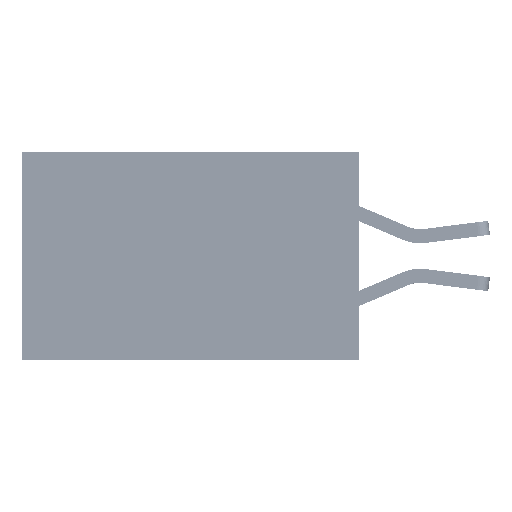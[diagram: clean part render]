
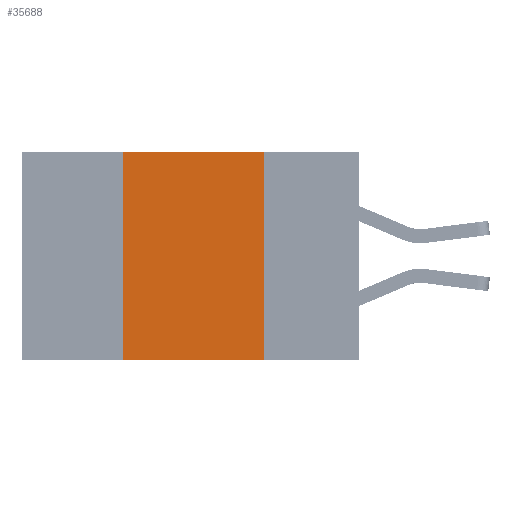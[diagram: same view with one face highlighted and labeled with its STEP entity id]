
A CAD part, left-side view. The second image highlights one B-rep face of the part: STEP entity #35688.
In plain terms, the highlighted planar face has unit normal (-1, 0, 0).
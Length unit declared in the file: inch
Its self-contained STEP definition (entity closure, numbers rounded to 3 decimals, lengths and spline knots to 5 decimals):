
#86 = VERTEX_POINT ( 'NONE', #17594 ) ;
#733 = DIRECTION ( 'NONE',  ( 0., -1., 0. ) ) ;
#2253 = LINE ( 'NONE', #8160, #23089 ) ;
#2528 = DIRECTION ( 'NONE',  ( 0., -1., 0. ) ) ;
#2641 = LINE ( 'NONE', #4090, #31487 ) ;
#4090 = CARTESIAN_POINT ( 'NONE',  ( 0., 0.6, -0.37 ) ) ;
#6305 = CARTESIAN_POINT ( 'NONE',  ( 0., 0.42, 0. ) ) ;
#6526 = VERTEX_POINT ( 'NONE', #41437 ) ;
#7997 = DIRECTION ( 'NONE',  ( 0., 0., 1. ) ) ;
#8160 = CARTESIAN_POINT ( 'NONE',  ( 0., 0.42, 0. ) ) ;
#9277 = ORIENTED_EDGE ( 'NONE', *, *, #33306, .F. ) ;
#9421 = CARTESIAN_POINT ( 'NONE',  ( 0., 0.17, 0. ) ) ;
#16019 = VECTOR ( 'NONE', #2528, 39.37008 ) ;
#17594 = CARTESIAN_POINT ( 'NONE',  ( 0., 0.17, -0.37 ) ) ;
#19320 = ORIENTED_EDGE ( 'NONE', *, *, #22238, .T. ) ;
#21200 = LINE ( 'NONE', #46892, #16019 ) ;
#21362 = FACE_OUTER_BOUND ( 'NONE', #26113, .T. ) ;
#21609 = DIRECTION ( 'NONE',  ( 1., 0., 0. ) ) ;
#21964 = EDGE_CURVE ( 'NONE', #31606, #43594, #21200, .T. ) ;
#22238 = EDGE_CURVE ( 'NONE', #6526, #86, #2641, .T. ) ;
#23089 = VECTOR ( 'NONE', #7997, 39.37008 ) ;
#25154 = DIRECTION ( 'NONE',  ( 0., 0., -1. ) ) ;
#25745 = AXIS2_PLACEMENT_3D ( 'NONE', #47211, #21609, #25154 ) ;
#26113 = EDGE_LOOP ( 'NONE', ( #9277, #46307, #41767, #19320 ) ) ;
#30201 = VECTOR ( 'NONE', #38652, 39.37008 ) ;
#31487 = VECTOR ( 'NONE', #733, 39.37008 ) ;
#31606 = VERTEX_POINT ( 'NONE', #6305 ) ;
#33306 = EDGE_CURVE ( 'NONE', #43594, #86, #38833, .T. ) ;
#35688 = ADVANCED_FACE ( 'NONE', ( #21362 ), #40568, .F. ) ;
#35713 = EDGE_CURVE ( 'NONE', #6526, #31606, #2253, .T. ) ;
#38652 = DIRECTION ( 'NONE',  ( 0., 0., -1. ) ) ;
#38833 = LINE ( 'NONE', #45151, #30201 ) ;
#40568 = PLANE ( 'NONE',  #25745 ) ;
#41437 = CARTESIAN_POINT ( 'NONE',  ( 0., 0.42, -0.37 ) ) ;
#41767 = ORIENTED_EDGE ( 'NONE', *, *, #35713, .F. ) ;
#43594 = VERTEX_POINT ( 'NONE', #9421 ) ;
#45151 = CARTESIAN_POINT ( 'NONE',  ( 0., 0.17, 0. ) ) ;
#46307 = ORIENTED_EDGE ( 'NONE', *, *, #21964, .F. ) ;
#46892 = CARTESIAN_POINT ( 'NONE',  ( 0., 0.6, 0. ) ) ;
#47211 = CARTESIAN_POINT ( 'NONE',  ( 0., 0.6, 0. ) ) ;
